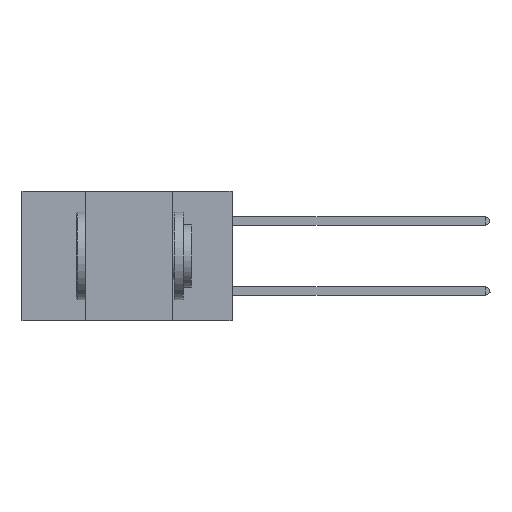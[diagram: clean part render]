
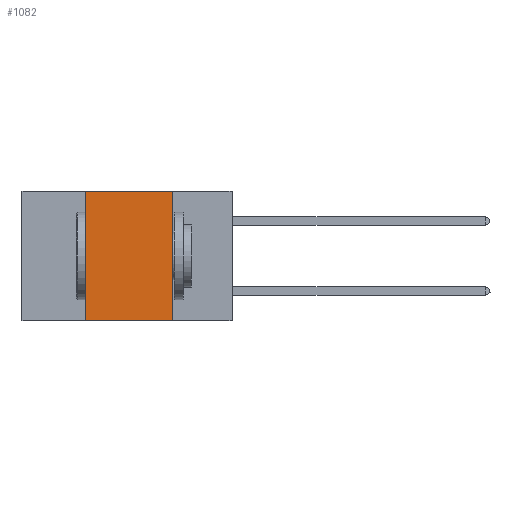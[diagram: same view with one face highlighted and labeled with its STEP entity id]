
A CAD part, left-side view. The second image highlights one B-rep face of the part: STEP entity #1082.
In plain terms, the highlighted planar face has unit normal (-1, 0, 0).
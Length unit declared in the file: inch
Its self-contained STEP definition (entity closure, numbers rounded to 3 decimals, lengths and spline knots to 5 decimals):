
#317 = CARTESIAN_POINT ( 'NONE',  ( 0., 0.42, -0.37 ) ) ;
#551 = EDGE_CURVE ( 'NONE', #8068, #3293, #4493, .T. ) ;
#1082 = ADVANCED_FACE ( 'NONE', ( #5343 ), #9813, .F. ) ;
#1433 = CARTESIAN_POINT ( 'NONE',  ( 0., 0.17, -0.37 ) ) ;
#2213 = LINE ( 'NONE', #3613, #12276 ) ;
#2559 = ORIENTED_EDGE ( 'NONE', *, *, #10017, .F. ) ;
#2729 = LINE ( 'NONE', #8208, #10178 ) ;
#3082 = EDGE_LOOP ( 'NONE', ( #2559, #5213, #8095, #10633 ) ) ;
#3293 = VERTEX_POINT ( 'NONE', #8654 ) ;
#3613 = CARTESIAN_POINT ( 'NONE',  ( 0., 0.6, -0.37 ) ) ;
#4196 = CARTESIAN_POINT ( 'NONE',  ( 0., 0.6, 0. ) ) ;
#4430 = DIRECTION ( 'NONE',  ( 0., 0., -1. ) ) ;
#4493 = LINE ( 'NONE', #5173, #9314 ) ;
#5103 = DIRECTION ( 'NONE',  ( 0., 0., 1. ) ) ;
#5173 = CARTESIAN_POINT ( 'NONE',  ( 0., 0.42, 0. ) ) ;
#5213 = ORIENTED_EDGE ( 'NONE', *, *, #11909, .F. ) ;
#5343 = FACE_OUTER_BOUND ( 'NONE', #3082, .T. ) ;
#6005 = EDGE_CURVE ( 'NONE', #8068, #9399, #2213, .T. ) ;
#6256 = DIRECTION ( 'NONE',  ( 0., -1., 0. ) ) ;
#6542 = VERTEX_POINT ( 'NONE', #12048 ) ;
#6561 = DIRECTION ( 'NONE',  ( 0., -1., 0. ) ) ;
#7656 = AXIS2_PLACEMENT_3D ( 'NONE', #4196, #9904, #4430 ) ;
#7772 = LINE ( 'NONE', #11970, #10282 ) ;
#8068 = VERTEX_POINT ( 'NONE', #317 ) ;
#8095 = ORIENTED_EDGE ( 'NONE', *, *, #551, .F. ) ;
#8208 = CARTESIAN_POINT ( 'NONE',  ( 0., 0.17, 0. ) ) ;
#8654 = CARTESIAN_POINT ( 'NONE',  ( 0., 0.42, 0. ) ) ;
#9165 = DIRECTION ( 'NONE',  ( 0., 0., -1. ) ) ;
#9314 = VECTOR ( 'NONE', #5103, 39.37008 ) ;
#9399 = VERTEX_POINT ( 'NONE', #1433 ) ;
#9813 = PLANE ( 'NONE',  #7656 ) ;
#9904 = DIRECTION ( 'NONE',  ( 1., 0., 0. ) ) ;
#10017 = EDGE_CURVE ( 'NONE', #6542, #9399, #2729, .T. ) ;
#10178 = VECTOR ( 'NONE', #9165, 39.37008 ) ;
#10282 = VECTOR ( 'NONE', #6256, 39.37008 ) ;
#10633 = ORIENTED_EDGE ( 'NONE', *, *, #6005, .T. ) ;
#11909 = EDGE_CURVE ( 'NONE', #3293, #6542, #7772, .T. ) ;
#11970 = CARTESIAN_POINT ( 'NONE',  ( 0., 0.6, 0. ) ) ;
#12048 = CARTESIAN_POINT ( 'NONE',  ( 0., 0.17, 0. ) ) ;
#12276 = VECTOR ( 'NONE', #6561, 39.37008 ) ;
